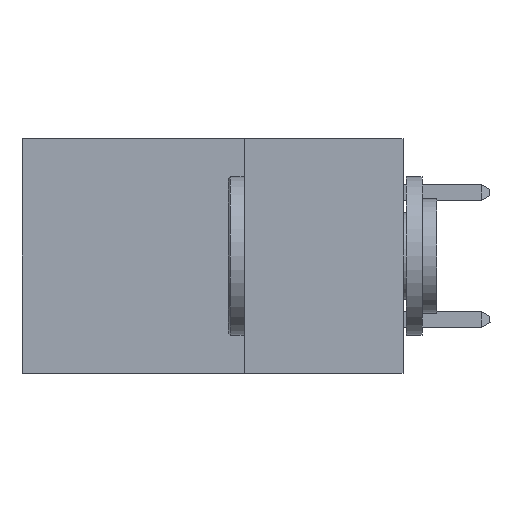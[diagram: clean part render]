
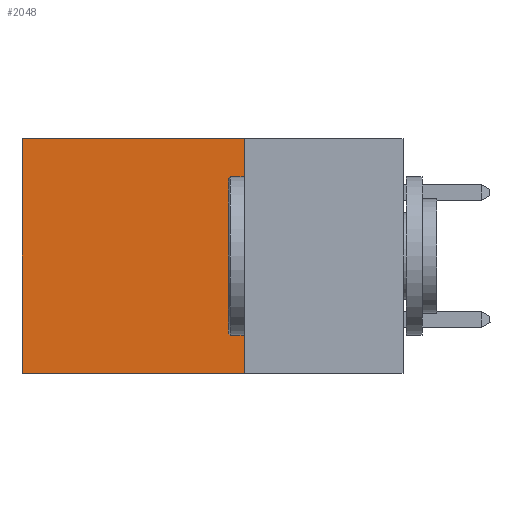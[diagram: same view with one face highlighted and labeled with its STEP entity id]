
A CAD part, left-side view. The second image highlights one B-rep face of the part: STEP entity #2048.
In plain terms, the highlighted planar face has unit normal (-1, 0, 0).
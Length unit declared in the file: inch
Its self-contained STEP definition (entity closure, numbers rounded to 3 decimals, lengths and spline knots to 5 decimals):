
#140 = CARTESIAN_POINT ( 'NONE',  ( 0.2875, 0.6, 0. ) ) ;
#205 = EDGE_LOOP ( 'NONE', ( #9112, #4460, #9181, #6261 ) ) ;
#214 = CARTESIAN_POINT ( 'NONE',  ( 0.2875, 0.25, 0. ) ) ;
#408 = CARTESIAN_POINT ( 'NONE',  ( 0.2875, 0.25, -0.37 ) ) ;
#442 = AXIS2_PLACEMENT_3D ( 'NONE', #2669, #2509, #997 ) ;
#469 = EDGE_CURVE ( 'NONE', #5203, #7681, #10510, .T. ) ;
#746 = EDGE_CURVE ( 'NONE', #8962, #3306, #3114, .T. ) ;
#849 = PLANE ( 'NONE',  #442 ) ;
#997 = DIRECTION ( 'NONE',  ( 0., 0., -1. ) ) ;
#1463 = DIRECTION ( 'NONE',  ( 0., 1., 0. ) ) ;
#1893 = FACE_OUTER_BOUND ( 'NONE', #205, .T. ) ;
#2048 = ADVANCED_FACE ( 'NONE', ( #1893 ), #849, .F. ) ;
#2162 = CARTESIAN_POINT ( 'NONE',  ( 0.2875, 0.25, -0.37 ) ) ;
#2509 = DIRECTION ( 'NONE',  ( 1., 0., 0. ) ) ;
#2669 = CARTESIAN_POINT ( 'NONE',  ( 0.2875, 0.25, 0. ) ) ;
#3114 = LINE ( 'NONE', #214, #10711 ) ;
#3306 = VERTEX_POINT ( 'NONE', #408 ) ;
#3615 = CARTESIAN_POINT ( 'NONE',  ( 0.2875, 0.6, 0. ) ) ;
#4221 = VECTOR ( 'NONE', #4390, 39.37008 ) ;
#4390 = DIRECTION ( 'NONE',  ( 0., 0., -1. ) ) ;
#4460 = ORIENTED_EDGE ( 'NONE', *, *, #5668, .F. ) ;
#4989 = VECTOR ( 'NONE', #1463, 39.37008 ) ;
#5203 = VERTEX_POINT ( 'NONE', #3615 ) ;
#5668 = EDGE_CURVE ( 'NONE', #3306, #7681, #10336, .T. ) ;
#6144 = CARTESIAN_POINT ( 'NONE',  ( 0.2875, 0.6, -0.37 ) ) ;
#6261 = ORIENTED_EDGE ( 'NONE', *, *, #7815, .T. ) ;
#6295 = LINE ( 'NONE', #9093, #4989 ) ;
#7681 = VERTEX_POINT ( 'NONE', #6144 ) ;
#7815 = EDGE_CURVE ( 'NONE', #8962, #5203, #6295, .T. ) ;
#8314 = CARTESIAN_POINT ( 'NONE',  ( 0.2875, 0.25, 0. ) ) ;
#8465 = DIRECTION ( 'NONE',  ( 0., 0., -1. ) ) ;
#8962 = VERTEX_POINT ( 'NONE', #8314 ) ;
#9093 = CARTESIAN_POINT ( 'NONE',  ( 0.2875, 0.25, 0. ) ) ;
#9112 = ORIENTED_EDGE ( 'NONE', *, *, #469, .T. ) ;
#9150 = VECTOR ( 'NONE', #9788, 39.37008 ) ;
#9181 = ORIENTED_EDGE ( 'NONE', *, *, #746, .F. ) ;
#9788 = DIRECTION ( 'NONE',  ( 0., 1., 0. ) ) ;
#10336 = LINE ( 'NONE', #2162, #9150 ) ;
#10510 = LINE ( 'NONE', #140, #4221 ) ;
#10711 = VECTOR ( 'NONE', #8465, 39.37008 ) ;
